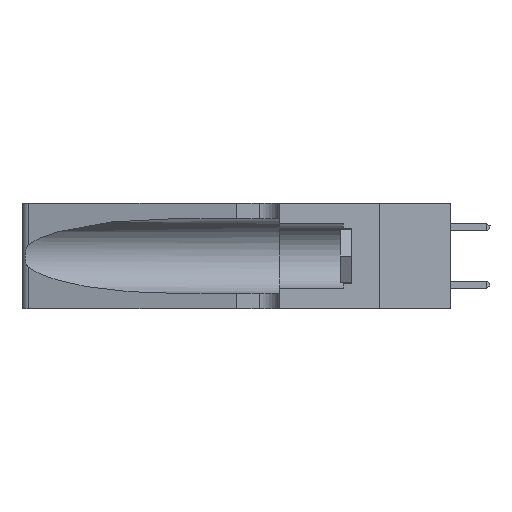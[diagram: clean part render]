
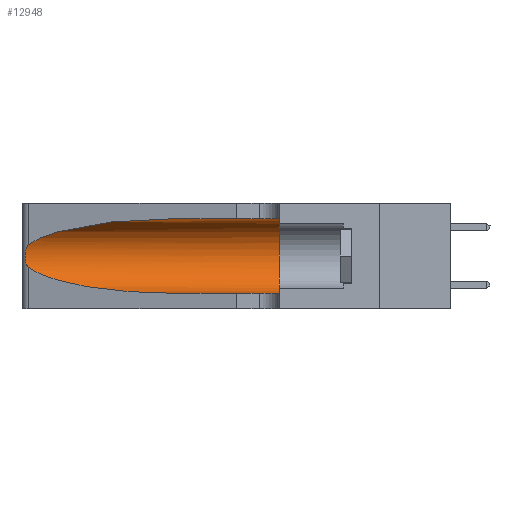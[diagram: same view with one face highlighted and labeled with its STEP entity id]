
A CAD part, left-side view. The second image highlights one B-rep face of the part: STEP entity #12948.
In plain terms, the highlighted cylindrical face has radius 3.308 mm (diameter 6.617 mm), a partial arc.
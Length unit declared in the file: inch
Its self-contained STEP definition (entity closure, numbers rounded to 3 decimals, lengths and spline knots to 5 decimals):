
#661 = CARTESIAN_POINT ( 'NONE',  ( 0.25639, 1.23184, 0.21858 ) ) ;
#724 = ORIENTED_EDGE ( 'NONE', *, *, #30350, .F. ) ;
#1229 = CYLINDRICAL_SURFACE ( 'NONE', #27392, 0.13025 ) ;
#1590 =( BOUNDED_CURVE ( )  B_SPLINE_CURVE ( 3, ( #4788, #32933, #20271, #4899 ),
 .UNSPECIFIED., .F., .F. ) 
 B_SPLINE_CURVE_WITH_KNOTS ( ( 4, 4 ),
 ( 3.44316, 4.71239 ),
 .UNSPECIFIED. ) 
 CURVE ( )  GEOMETRIC_REPRESENTATION_ITEM ( )  RATIONAL_B_SPLINE_CURVE ( ( 1., 0.87, 0.87, 1. ) ) 
 REPRESENTATION_ITEM ( '' )  );
#3284 = CARTESIAN_POINT ( 'NONE',  ( 0.25854, 1.2359, 0.20912 ) ) ;
#4400 = CARTESIAN_POINT ( 'NONE',  ( 0.1305, 0.35, 0.185 ) ) ;
#4788 = CARTESIAN_POINT ( 'NONE',  ( 0.25487, 1.22718, 0.14631 ) ) ;
#4899 = CARTESIAN_POINT ( 'NONE',  ( 0.1305, 0.72297, 0.05475 ) ) ;
#5918 = CARTESIAN_POINT ( 'NONE',  ( 0.26075, 1.23896, 0.19203 ) ) ;
#6310 = LINE ( 'NONE', #15068, #25939 ) ;
#6370 = DIRECTION ( 'NONE',  ( 0., -1., 0. ) ) ;
#7007 = DIRECTION ( 'NONE',  ( 0., 0., 1. ) ) ;
#7259 = AXIS2_PLACEMENT_3D ( 'NONE', #4400, #22353, #7007 ) ;
#7636 = EDGE_CURVE ( 'NONE', #33148, #8023, #8517, .T. ) ;
#7690 = CARTESIAN_POINT ( 'NONE',  ( 0.1305, 0.35, 0.05475 ) ) ;
#7713 = VECTOR ( 'NONE', #8894, 39.37008 ) ;
#8023 = VERTEX_POINT ( 'NONE', #15556 ) ;
#8253 = CARTESIAN_POINT ( 'NONE',  ( 0.1305, 0.72297, 0.05475 ) ) ;
#8517 = LINE ( 'NONE', #16589, #7713 ) ;
#8518 = CARTESIAN_POINT ( 'NONE',  ( 0.26017, 1.23833, 0.17102 ) ) ;
#8894 = DIRECTION ( 'NONE',  ( 0., -1., 0. ) ) ;
#8964 = FACE_OUTER_BOUND ( 'NONE', #29171, .T. ) ;
#8983 = DIRECTION ( 'NONE',  ( 0., 0., -1. ) ) ;
#11056 = CARTESIAN_POINT ( 'NONE',  ( 0.25487, 1.22718, 0.14631 ) ) ;
#11092 = CARTESIAN_POINT ( 'NONE',  ( 0.25789, 1.23486, 0.15765 ) ) ;
#12948 = ADVANCED_FACE ( 'NONE', ( #8964 ), #1229, .F. ) ;
#13184 = CARTESIAN_POINT ( 'NONE',  ( 0.25487, 1.22718, 0.22369 ) ) ;
#13522 = CARTESIAN_POINT ( 'NONE',  ( 0.25487, 1.22718, 0.22369 ) ) ;
#13576 = B_SPLINE_CURVE_WITH_KNOTS ( 'NONE', 3,
 ( #13522, #28741, #661, #18694, #3284, #21255, #5918, #23850, #8518, #26391, #11092, #28956, #13624, #31495 ),
 .UNSPECIFIED., .F., .F.,
 ( 4, 2, 2, 2, 2, 2, 4 ),
 ( 0., 0.00027, 0.00053, 0.00107, 0.0016, 0.00187, 0.00214 ),
 .UNSPECIFIED. ) ;
#13624 = CARTESIAN_POINT ( 'NONE',  ( 0.25555, 1.22993, 0.14849 ) ) ;
#13982 = CARTESIAN_POINT ( 'NONE',  ( 0.1305, 1.61858, 0.185 ) ) ;
#13983 = VERTEX_POINT ( 'NONE', #7690 ) ;
#15068 = CARTESIAN_POINT ( 'NONE',  ( 0.1305, 1.61858, 0.05475 ) ) ;
#15556 = CARTESIAN_POINT ( 'NONE',  ( 0.1305, 0.35, 0.31525 ) ) ;
#16589 = CARTESIAN_POINT ( 'NONE',  ( 0.1305, 1.61858, 0.31525 ) ) ;
#17381 = VERTEX_POINT ( 'NONE', #26882 ) ;
#17637 = DIRECTION ( 'NONE',  ( 0., -1., 0. ) ) ;
#17677 = CIRCLE ( 'NONE', #7259, 0.13025 ) ;
#17925 = EDGE_CURVE ( 'NONE', #17381, #29391, #13576, .T. ) ;
#18234 = CARTESIAN_POINT ( 'NONE',  ( 0.18966, 0.96281, 0.31525 ) ) ;
#18694 = CARTESIAN_POINT ( 'NONE',  ( 0.25787, 1.23484, 0.2124 ) ) ;
#19616 = ORIENTED_EDGE ( 'NONE', *, *, #17925, .T. ) ;
#19881 = ORIENTED_EDGE ( 'NONE', *, *, #21353, .T. ) ;
#20271 = CARTESIAN_POINT ( 'NONE',  ( 0.18966, 0.96281, 0.05475 ) ) ;
#21255 = CARTESIAN_POINT ( 'NONE',  ( 0.26018, 1.23835, 0.19895 ) ) ;
#21353 = EDGE_CURVE ( 'NONE', #29904, #13983, #6310, .T. ) ;
#22353 = DIRECTION ( 'NONE',  ( 0., 1., 0. ) ) ;
#23393 = CARTESIAN_POINT ( 'NONE',  ( 0.1305, 0.72297, 0.31525 ) ) ;
#23850 = CARTESIAN_POINT ( 'NONE',  ( 0.26075, 1.23896, 0.178 ) ) ;
#24228 = ORIENTED_EDGE ( 'NONE', *, *, #7636, .F. ) ;
#25037 = EDGE_CURVE ( 'NONE', #29391, #29904, #1590, .T. ) ;
#25153 = EDGE_CURVE ( 'NONE', #33148, #17381, #28968, .T. ) ;
#25437 = ORIENTED_EDGE ( 'NONE', *, *, #25037, .T. ) ;
#25856 = CARTESIAN_POINT ( 'NONE',  ( 0.1305, 0.72297, 0.31525 ) ) ;
#25939 = VECTOR ( 'NONE', #17637, 39.37008 ) ;
#26391 = CARTESIAN_POINT ( 'NONE',  ( 0.25856, 1.23593, 0.16098 ) ) ;
#26882 = CARTESIAN_POINT ( 'NONE',  ( 0.25487, 1.22718, 0.22369 ) ) ;
#27392 = AXIS2_PLACEMENT_3D ( 'NONE', #13982, #6370, #8983 ) ;
#28507 = CARTESIAN_POINT ( 'NONE',  ( 0.2373, 1.15595, 0.28018 ) ) ;
#28741 = CARTESIAN_POINT ( 'NONE',  ( 0.25555, 1.22994, 0.2215 ) ) ;
#28956 = CARTESIAN_POINT ( 'NONE',  ( 0.25639, 1.23186, 0.15144 ) ) ;
#28968 =( BOUNDED_CURVE ( )  B_SPLINE_CURVE ( 3, ( #23393, #18234, #28507, #13184 ),
 .UNSPECIFIED., .F., .F. ) 
 B_SPLINE_CURVE_WITH_KNOTS ( ( 4, 4 ),
 ( 1.5708, 2.84003 ),
 .UNSPECIFIED. ) 
 CURVE ( )  GEOMETRIC_REPRESENTATION_ITEM ( )  RATIONAL_B_SPLINE_CURVE ( ( 1., 0.87, 0.87, 1. ) ) 
 REPRESENTATION_ITEM ( '' )  );
#29171 = EDGE_LOOP ( 'NONE', ( #31380, #19616, #25437, #19881, #724, #24228 ) ) ;
#29391 = VERTEX_POINT ( 'NONE', #11056 ) ;
#29904 = VERTEX_POINT ( 'NONE', #8253 ) ;
#30350 = EDGE_CURVE ( 'NONE', #8023, #13983, #17677, .T. ) ;
#31380 = ORIENTED_EDGE ( 'NONE', *, *, #25153, .T. ) ;
#31495 = CARTESIAN_POINT ( 'NONE',  ( 0.25487, 1.22718, 0.14631 ) ) ;
#32933 = CARTESIAN_POINT ( 'NONE',  ( 0.2373, 1.15595, 0.08982 ) ) ;
#33148 = VERTEX_POINT ( 'NONE', #25856 ) ;
